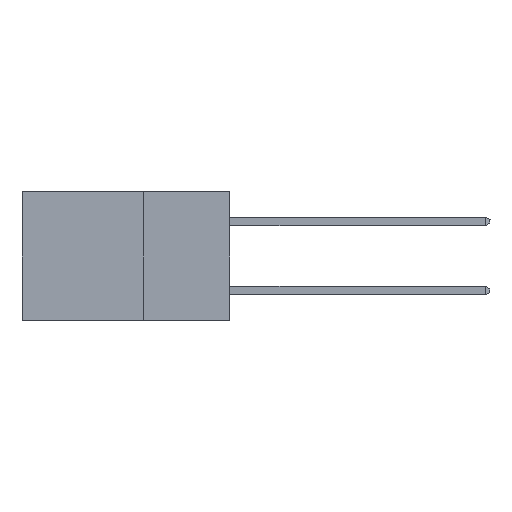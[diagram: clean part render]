
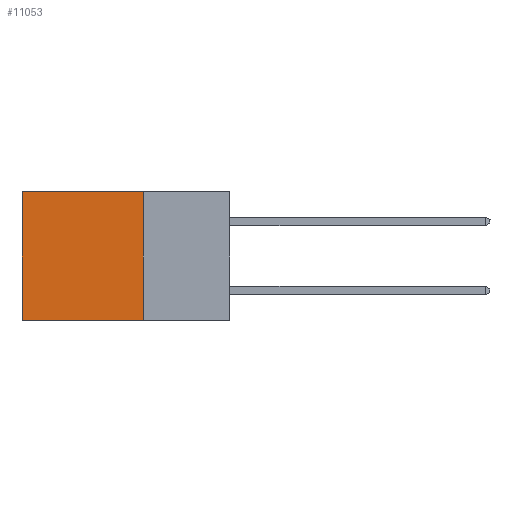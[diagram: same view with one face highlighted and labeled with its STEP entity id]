
A CAD part, left-side view. The second image highlights one B-rep face of the part: STEP entity #11053.
In plain terms, the highlighted planar face has unit normal (-1, 0, 0).
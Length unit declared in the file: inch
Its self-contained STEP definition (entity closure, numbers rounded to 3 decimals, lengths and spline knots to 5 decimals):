
#39 = VECTOR ( 'NONE', #3469, 39.37008 ) ;
#403 = AXIS2_PLACEMENT_3D ( 'NONE', #12553, #14353, #14237 ) ;
#439 = VERTEX_POINT ( 'NONE', #6275 ) ;
#1541 = EDGE_CURVE ( 'NONE', #16610, #2333, #5161, .T. ) ;
#2194 = PLANE ( 'NONE',  #403 ) ;
#2333 = VERTEX_POINT ( 'NONE', #18148 ) ;
#3469 = DIRECTION ( 'NONE',  ( 0., 1., 0. ) ) ;
#3829 = EDGE_CURVE ( 'NONE', #439, #16610, #11002, .T. ) ;
#3862 = CARTESIAN_POINT ( 'NONE',  ( 0.2615, 0.25, -0.37 ) ) ;
#3943 = DIRECTION ( 'NONE',  ( 0., 1., 0. ) ) ;
#4400 = VERTEX_POINT ( 'NONE', #7198 ) ;
#4654 = VECTOR ( 'NONE', #5961, 39.37008 ) ;
#5161 = LINE ( 'NONE', #12095, #39 ) ;
#5510 = ORIENTED_EDGE ( 'NONE', *, *, #18398, .T. ) ;
#5666 = ORIENTED_EDGE ( 'NONE', *, *, #1541, .F. ) ;
#5961 = DIRECTION ( 'NONE',  ( 0., 0., -1. ) ) ;
#6275 = CARTESIAN_POINT ( 'NONE',  ( 0.2615, 0.25, 0. ) ) ;
#7198 = CARTESIAN_POINT ( 'NONE',  ( 0.2615, 0.6, 0. ) ) ;
#7940 = VECTOR ( 'NONE', #3943, 39.37008 ) ;
#9016 = FACE_OUTER_BOUND ( 'NONE', #20861, .T. ) ;
#10972 = CARTESIAN_POINT ( 'NONE',  ( 0.2615, 0.25, -0.37 ) ) ;
#11002 = LINE ( 'NONE', #3862, #12729 ) ;
#11053 = ADVANCED_FACE ( 'NONE', ( #9016 ), #2194, .F. ) ;
#12095 = CARTESIAN_POINT ( 'NONE',  ( 0.2615, 0.25, -0.37 ) ) ;
#12553 = CARTESIAN_POINT ( 'NONE',  ( 0.2615, 0.25, -0.37 ) ) ;
#12698 = DIRECTION ( 'NONE',  ( 0., 0., -1. ) ) ;
#12729 = VECTOR ( 'NONE', #12698, 39.37008 ) ;
#14237 = DIRECTION ( 'NONE',  ( 0., 0., -1. ) ) ;
#14353 = DIRECTION ( 'NONE',  ( 1., 0., 0. ) ) ;
#16129 = ORIENTED_EDGE ( 'NONE', *, *, #20740, .T. ) ;
#16172 = ORIENTED_EDGE ( 'NONE', *, *, #3829, .F. ) ;
#16610 = VERTEX_POINT ( 'NONE', #10972 ) ;
#16702 = LINE ( 'NONE', #21685, #4654 ) ;
#18148 = CARTESIAN_POINT ( 'NONE',  ( 0.2615, 0.6, -0.37 ) ) ;
#18398 = EDGE_CURVE ( 'NONE', #439, #4400, #19470, .T. ) ;
#19470 = LINE ( 'NONE', #19864, #7940 ) ;
#19864 = CARTESIAN_POINT ( 'NONE',  ( 0.2615, 0.25, 0. ) ) ;
#20740 = EDGE_CURVE ( 'NONE', #4400, #2333, #16702, .T. ) ;
#20861 = EDGE_LOOP ( 'NONE', ( #16129, #5666, #16172, #5510 ) ) ;
#21685 = CARTESIAN_POINT ( 'NONE',  ( 0.2615, 0.6, -0.37 ) ) ;
